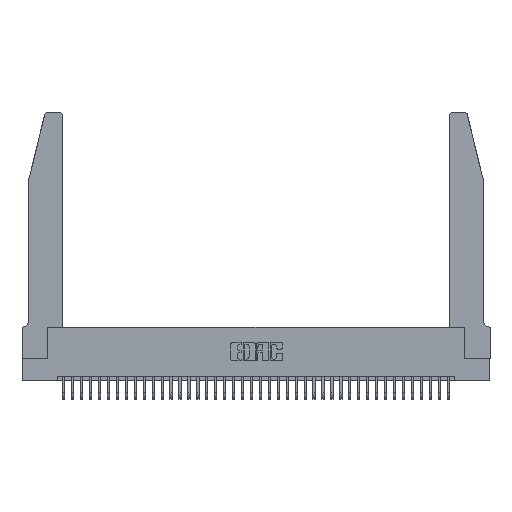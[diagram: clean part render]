
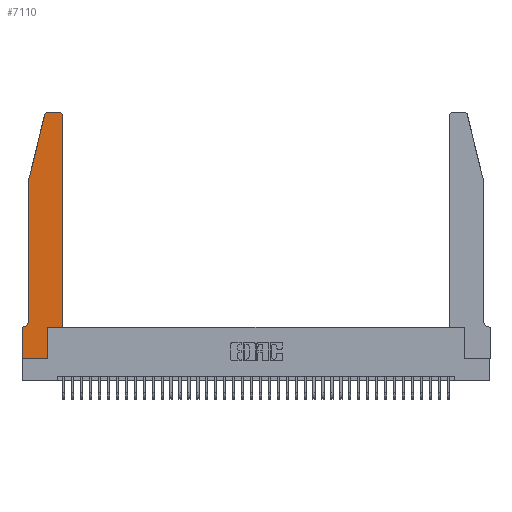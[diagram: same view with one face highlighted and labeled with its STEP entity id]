
A CAD part, top view. The second image highlights one B-rep face of the part: STEP entity #7110.
In plain terms, the highlighted planar face has unit normal (0, 0, 1).
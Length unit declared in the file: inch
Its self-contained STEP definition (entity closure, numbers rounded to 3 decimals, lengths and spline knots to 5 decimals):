
#496 = CARTESIAN_POINT ( 'NONE',  ( 0.284, 2.75, 0.37 ) ) ;
#767 = CARTESIAN_POINT ( 'NONE',  ( 0., 0., 0.37 ) ) ;
#1061 = AXIS2_PLACEMENT_3D ( 'NONE', #18772, #29511, #4625 ) ;
#1432 = CARTESIAN_POINT ( 'NONE',  ( 0.4505, 0.35, 0.37 ) ) ;
#1551 = CARTESIAN_POINT ( 'NONE',  ( 0.0755, 2., 0.37 ) ) ;
#1939 = LINE ( 'NONE', #3184, #24580 ) ;
#2126 = CARTESIAN_POINT ( 'NONE',  ( 0.4505, 2.72, 0.37 ) ) ;
#3184 = CARTESIAN_POINT ( 'NONE',  ( 0.2605, 2.75, 0.37 ) ) ;
#3630 = DIRECTION ( 'NONE',  ( 1., 0., 0. ) ) ;
#4625 = DIRECTION ( 'NONE',  ( -1., 0., 0. ) ) ;
#5083 = EDGE_CURVE ( 'NONE', #8848, #38212, #27723, .T. ) ;
#5232 = EDGE_CURVE ( 'NONE', #5893, #8848, #15950, .T. ) ;
#5704 = ORIENTED_EDGE ( 'NONE', *, *, #31696, .T. ) ;
#5893 = VERTEX_POINT ( 'NONE', #35003 ) ;
#6824 = DIRECTION ( 'NONE',  ( 0., 0., 1. ) ) ;
#6970 = VECTOR ( 'NONE', #34606, 39.37008 ) ;
#7110 = ADVANCED_FACE ( 'NONE', ( #15839 ), #7176, .T. ) ;
#7176 = PLANE ( 'NONE',  #26901 ) ;
#7283 = CARTESIAN_POINT ( 'NONE',  ( 0.4205, 2.75, 0.37 ) ) ;
#7377 = DIRECTION ( 'NONE',  ( -0.239, -0.971, 0. ) ) ;
#7534 = CARTESIAN_POINT ( 'NONE',  ( 0.2865, 0., 0.37 ) ) ;
#7825 = EDGE_CURVE ( 'NONE', #39888, #23748, #1939, .T. ) ;
#8646 = AXIS2_PLACEMENT_3D ( 'NONE', #25650, #6824, #10019 ) ;
#8821 = EDGE_LOOP ( 'NONE', ( #26889, #36764, #36302, #23961, #18777, #36775, #35485, #23322, #5704, #34716, #31120, #18876 ) ) ;
#8848 = VERTEX_POINT ( 'NONE', #18487 ) ;
#10018 = CIRCLE ( 'NONE', #8646, 0.03 ) ;
#10019 = DIRECTION ( 'NONE',  ( 1., 0., 0. ) ) ;
#10093 = DIRECTION ( 'NONE',  ( 0., 0., 1. ) ) ;
#11062 = EDGE_CURVE ( 'NONE', #17911, #36822, #24083, .T. ) ;
#11566 = EDGE_CURVE ( 'NONE', #16452, #34232, #20636, .T. ) ;
#11618 = CARTESIAN_POINT ( 'NONE',  ( 0.0055, 0.35, 0.37 ) ) ;
#14077 = VERTEX_POINT ( 'NONE', #26472 ) ;
#15352 = DIRECTION ( 'NONE',  ( -1., 0., 0. ) ) ;
#15557 = LINE ( 'NONE', #27355, #30329 ) ;
#15583 = VERTEX_POINT ( 'NONE', #11618 ) ;
#15839 = FACE_OUTER_BOUND ( 'NONE', #8821, .T. ) ;
#15950 = LINE ( 'NONE', #1432, #23274 ) ;
#16452 = VERTEX_POINT ( 'NONE', #33003 ) ;
#17911 = VERTEX_POINT ( 'NONE', #19161 ) ;
#18042 = CARTESIAN_POINT ( 'NONE',  ( 0., 0.35, 0.37 ) ) ;
#18447 = LINE ( 'NONE', #30985, #21873 ) ;
#18487 = CARTESIAN_POINT ( 'NONE',  ( 0.4505, 0.35, 0.37 ) ) ;
#18772 = CARTESIAN_POINT ( 'NONE',  ( 0.0055, 0.42, 0.37 ) ) ;
#18777 = ORIENTED_EDGE ( 'NONE', *, *, #22465, .T. ) ;
#18876 = ORIENTED_EDGE ( 'NONE', *, *, #21222, .T. ) ;
#19161 = CARTESIAN_POINT ( 'NONE',  ( 0., 0., 0.37 ) ) ;
#19451 = EDGE_CURVE ( 'NONE', #15583, #29825, #15557, .T. ) ;
#20019 = LINE ( 'NONE', #20567, #31863 ) ;
#20499 = CARTESIAN_POINT ( 'NONE',  ( 0.284, 2.72, 0.37 ) ) ;
#20567 = CARTESIAN_POINT ( 'NONE',  ( 0.2865, 0.35, 0.37 ) ) ;
#20636 = LINE ( 'NONE', #23803, #39332 ) ;
#21046 = AXIS2_PLACEMENT_3D ( 'NONE', #20499, #32767, #32895 ) ;
#21222 = EDGE_CURVE ( 'NONE', #38212, #39888, #10018, .T. ) ;
#21873 = VECTOR ( 'NONE', #33684, 39.37008 ) ;
#22078 = EDGE_CURVE ( 'NONE', #23748, #16452, #34926, .T. ) ;
#22465 = EDGE_CURVE ( 'NONE', #14077, #15583, #31496, .T. ) ;
#23274 = VECTOR ( 'NONE', #39618, 39.37008 ) ;
#23322 = ORIENTED_EDGE ( 'NONE', *, *, #11062, .T. ) ;
#23721 = DIRECTION ( 'NONE',  ( 0., 1., 0. ) ) ;
#23748 = VERTEX_POINT ( 'NONE', #496 ) ;
#23803 = CARTESIAN_POINT ( 'NONE',  ( 0.0755, 2., 0.37 ) ) ;
#23961 = ORIENTED_EDGE ( 'NONE', *, *, #25933, .T. ) ;
#24083 = LINE ( 'NONE', #767, #37854 ) ;
#24580 = VECTOR ( 'NONE', #15352, 39.37008 ) ;
#25650 = CARTESIAN_POINT ( 'NONE',  ( 0.4205, 2.72, 0.37 ) ) ;
#25933 = EDGE_CURVE ( 'NONE', #34232, #14077, #18447, .T. ) ;
#26472 = CARTESIAN_POINT ( 'NONE',  ( 0.0755, 0.42, 0.37 ) ) ;
#26835 = CARTESIAN_POINT ( 'NONE',  ( 0., 0.35, 0.37 ) ) ;
#26889 = ORIENTED_EDGE ( 'NONE', *, *, #7825, .T. ) ;
#26901 = AXIS2_PLACEMENT_3D ( 'NONE', #26835, #10093, #35208 ) ;
#27355 = CARTESIAN_POINT ( 'NONE',  ( 0.0755, 0.35, 0.37 ) ) ;
#27723 = LINE ( 'NONE', #31275, #36566 ) ;
#28575 = CARTESIAN_POINT ( 'NONE',  ( 0., 0., 0.37 ) ) ;
#29511 = DIRECTION ( 'NONE',  ( 0., 0., -1. ) ) ;
#29825 = VERTEX_POINT ( 'NONE', #18042 ) ;
#30329 = VECTOR ( 'NONE', #33662, 39.37008 ) ;
#30985 = CARTESIAN_POINT ( 'NONE',  ( 0.0755, 2., 0.37 ) ) ;
#31008 = DIRECTION ( 'NONE',  ( 0., 1., 0. ) ) ;
#31120 = ORIENTED_EDGE ( 'NONE', *, *, #5083, .T. ) ;
#31275 = CARTESIAN_POINT ( 'NONE',  ( 0.4505, 0.35, 0.37 ) ) ;
#31496 = CIRCLE ( 'NONE', #1061, 0.07 ) ;
#31696 = EDGE_CURVE ( 'NONE', #36822, #5893, #20019, .T. ) ;
#31863 = VECTOR ( 'NONE', #23721, 39.37008 ) ;
#32767 = DIRECTION ( 'NONE',  ( 0., 0., 1. ) ) ;
#32895 = DIRECTION ( 'NONE',  ( 1., 0., 0. ) ) ;
#33003 = CARTESIAN_POINT ( 'NONE',  ( 0.25487, 2.72718, 0.37 ) ) ;
#33662 = DIRECTION ( 'NONE',  ( -1., 0., 0. ) ) ;
#33684 = DIRECTION ( 'NONE',  ( 0., -1., 0. ) ) ;
#34232 = VERTEX_POINT ( 'NONE', #1551 ) ;
#34606 = DIRECTION ( 'NONE',  ( 0., -1., 0. ) ) ;
#34716 = ORIENTED_EDGE ( 'NONE', *, *, #5232, .T. ) ;
#34723 = EDGE_CURVE ( 'NONE', #29825, #17911, #39913, .T. ) ;
#34926 = CIRCLE ( 'NONE', #21046, 0.03 ) ;
#35003 = CARTESIAN_POINT ( 'NONE',  ( 0.2865, 0.35, 0.37 ) ) ;
#35208 = DIRECTION ( 'NONE',  ( 1., 0., 0. ) ) ;
#35485 = ORIENTED_EDGE ( 'NONE', *, *, #34723, .T. ) ;
#36302 = ORIENTED_EDGE ( 'NONE', *, *, #11566, .T. ) ;
#36566 = VECTOR ( 'NONE', #31008, 39.37008 ) ;
#36764 = ORIENTED_EDGE ( 'NONE', *, *, #22078, .T. ) ;
#36775 = ORIENTED_EDGE ( 'NONE', *, *, #19451, .T. ) ;
#36822 = VERTEX_POINT ( 'NONE', #7534 ) ;
#37854 = VECTOR ( 'NONE', #3630, 39.37008 ) ;
#38212 = VERTEX_POINT ( 'NONE', #2126 ) ;
#39332 = VECTOR ( 'NONE', #7377, 39.37008 ) ;
#39618 = DIRECTION ( 'NONE',  ( 1., 0., 0. ) ) ;
#39888 = VERTEX_POINT ( 'NONE', #7283 ) ;
#39913 = LINE ( 'NONE', #28575, #6970 ) ;
